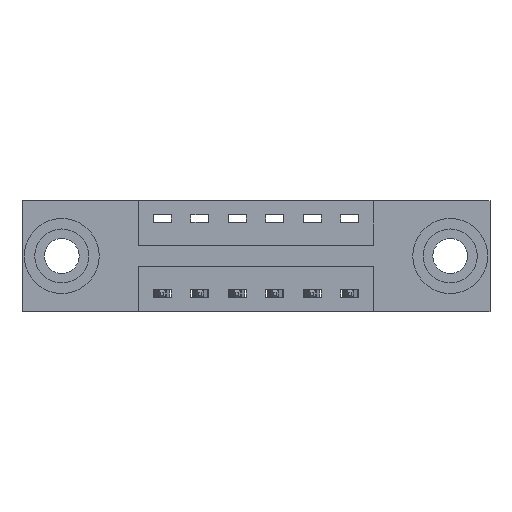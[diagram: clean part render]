
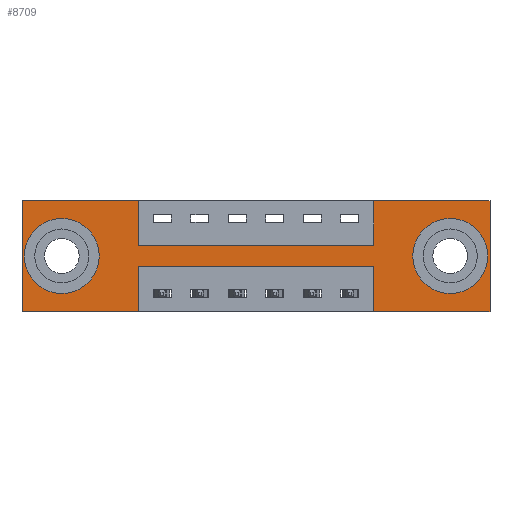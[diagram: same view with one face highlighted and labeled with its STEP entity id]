
A CAD part, front view. The second image highlights one B-rep face of the part: STEP entity #8709.
In plain terms, the highlighted planar face has unit normal (0, -1, 0).
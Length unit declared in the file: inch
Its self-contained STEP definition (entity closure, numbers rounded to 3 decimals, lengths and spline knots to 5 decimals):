
#26 = LINE ( 'NONE', #4180, #5524 ) ;
#77 = EDGE_LOOP ( 'NONE', ( #3163, #3465 ) ) ;
#123 = VERTEX_POINT ( 'NONE', #2344 ) ;
#150 = EDGE_CURVE ( 'NONE', #1095, #9016, #529, .T. ) ;
#191 = CARTESIAN_POINT ( 'NONE',  ( 0., 0., -0.37 ) ) ;
#247 = EDGE_CURVE ( 'NONE', #3096, #1057, #26, .T. ) ;
#474 = CARTESIAN_POINT ( 'NONE',  ( 0.1325, 0., -0.185 ) ) ;
#517 = EDGE_CURVE ( 'NONE', #7520, #5748, #3592, .T. ) ;
#529 = CIRCLE ( 'NONE', #5167, 0.078 ) ;
#539 = ORIENTED_EDGE ( 'NONE', *, *, #517, .F. ) ;
#695 = VECTOR ( 'NONE', #3651, 39.37008 ) ;
#874 = DIRECTION ( 'NONE',  ( 0., 0., 1. ) ) ;
#974 = DIRECTION ( 'NONE',  ( 1., 0., 0. ) ) ;
#1005 = ORIENTED_EDGE ( 'NONE', *, *, #8108, .F. ) ;
#1057 = VERTEX_POINT ( 'NONE', #3721 ) ;
#1066 = DIRECTION ( 'NONE',  ( -1., 0., 0. ) ) ;
#1095 = VERTEX_POINT ( 'NONE', #3238 ) ;
#1107 = LINE ( 'NONE', #4271, #6540 ) ;
#1227 = DIRECTION ( 'NONE',  ( 0., 0., 1. ) ) ;
#1295 = VERTEX_POINT ( 'NONE', #2294 ) ;
#1296 = CARTESIAN_POINT ( 'NONE',  ( 0.1325, 0., -0.263 ) ) ;
#1390 = EDGE_CURVE ( 'NONE', #1295, #7130, #1107, .T. ) ;
#1508 = CIRCLE ( 'NONE', #5842, 0.078 ) ;
#1532 = VERTEX_POINT ( 'NONE', #8157 ) ;
#1543 = CARTESIAN_POINT ( 'NONE',  ( 1.1725, 0., 0. ) ) ;
#1601 = EDGE_CURVE ( 'NONE', #4266, #6499, #2909, .T. ) ;
#1611 = FACE_OUTER_BOUND ( 'NONE', #5340, .T. ) ;
#1749 = EDGE_CURVE ( 'NONE', #1057, #4266, #2249, .T. ) ;
#1754 = AXIS2_PLACEMENT_3D ( 'NONE', #3625, #8518, #4333 ) ;
#1825 = AXIS2_PLACEMENT_3D ( 'NONE', #191, #7342, #3143 ) ;
#1878 = DIRECTION ( 'NONE',  ( 1., 0., 0. ) ) ;
#1910 = CARTESIAN_POINT ( 'NONE',  ( 1.4275, 0., -0.185 ) ) ;
#1961 = VECTOR ( 'NONE', #974, 39.37008 ) ;
#2055 = VERTEX_POINT ( 'NONE', #6461 ) ;
#2122 = VECTOR ( 'NONE', #874, 39.37008 ) ;
#2213 = CARTESIAN_POINT ( 'NONE',  ( 0.3875, 0., -0.22 ) ) ;
#2249 = LINE ( 'NONE', #6686, #6193 ) ;
#2294 = CARTESIAN_POINT ( 'NONE',  ( 0.3875, 0., -0.22 ) ) ;
#2318 = EDGE_CURVE ( 'NONE', #9016, #1095, #2347, .T. ) ;
#2344 = CARTESIAN_POINT ( 'NONE',  ( 0.3875, 0., -0.15 ) ) ;
#2347 = CIRCLE ( 'NONE', #3344, 0.078 ) ;
#2526 = VECTOR ( 'NONE', #1066, 39.37008 ) ;
#2622 = DIRECTION ( 'NONE',  ( 0., 0., -1. ) ) ;
#2624 = EDGE_CURVE ( 'NONE', #1532, #123, #5046, .T. ) ;
#2713 = ORIENTED_EDGE ( 'NONE', *, *, #7315, .F. ) ;
#2909 = LINE ( 'NONE', #4907, #8513 ) ;
#2913 = DIRECTION ( 'NONE',  ( -1., 0., 0. ) ) ;
#2933 = CARTESIAN_POINT ( 'NONE',  ( 0., 0., 0. ) ) ;
#2988 = DIRECTION ( 'NONE',  ( 0., 0., -1. ) ) ;
#3096 = VERTEX_POINT ( 'NONE', #1543 ) ;
#3143 = DIRECTION ( 'NONE',  ( 0., 0., -1. ) ) ;
#3163 = ORIENTED_EDGE ( 'NONE', *, *, #4598, .T. ) ;
#3238 = CARTESIAN_POINT ( 'NONE',  ( 0.1325, 0., -0.107 ) ) ;
#3278 = VECTOR ( 'NONE', #4980, 39.37008 ) ;
#3307 = DIRECTION ( 'NONE',  ( 0., 0., 1. ) ) ;
#3344 = AXIS2_PLACEMENT_3D ( 'NONE', #474, #5439, #1227 ) ;
#3366 = ORIENTED_EDGE ( 'NONE', *, *, #150, .T. ) ;
#3465 = ORIENTED_EDGE ( 'NONE', *, *, #7281, .T. ) ;
#3592 = LINE ( 'NONE', #8836, #6770 ) ;
#3612 = ORIENTED_EDGE ( 'NONE', *, *, #1749, .F. ) ;
#3625 = CARTESIAN_POINT ( 'NONE',  ( 1.4275, 0., -0.185 ) ) ;
#3651 = DIRECTION ( 'NONE',  ( 1., 0., 0. ) ) ;
#3721 = CARTESIAN_POINT ( 'NONE',  ( 1.56, 0., 0. ) ) ;
#3775 = LINE ( 'NONE', #5114, #2122 ) ;
#3810 = CARTESIAN_POINT ( 'NONE',  ( 1.1725, 0., -0.37 ) ) ;
#3862 = ORIENTED_EDGE ( 'NONE', *, *, #9186, .F. ) ;
#4157 = ORIENTED_EDGE ( 'NONE', *, *, #2318, .T. ) ;
#4180 = CARTESIAN_POINT ( 'NONE',  ( 0., 0., 0. ) ) ;
#4266 = VERTEX_POINT ( 'NONE', #4353 ) ;
#4271 = CARTESIAN_POINT ( 'NONE',  ( 0.3875, 0., -0.37 ) ) ;
#4313 = CARTESIAN_POINT ( 'NONE',  ( 1.1725, 0., -0.22 ) ) ;
#4333 = DIRECTION ( 'NONE',  ( 0., 0., -1. ) ) ;
#4353 = CARTESIAN_POINT ( 'NONE',  ( 1.56, 0., -0.37 ) ) ;
#4598 = EDGE_CURVE ( 'NONE', #2055, #6014, #1508, .T. ) ;
#4688 = VERTEX_POINT ( 'NONE', #6932 ) ;
#4744 = VECTOR ( 'NONE', #5171, 39.37008 ) ;
#4834 = CARTESIAN_POINT ( 'NONE',  ( 0.3875, 0., -0.37 ) ) ;
#4858 = VECTOR ( 'NONE', #5798, 39.37008 ) ;
#4907 = CARTESIAN_POINT ( 'NONE',  ( 0., 0., -0.37 ) ) ;
#4967 = EDGE_CURVE ( 'NONE', #123, #4688, #5438, .T. ) ;
#4980 = DIRECTION ( 'NONE',  ( -1., 0., 0. ) ) ;
#5046 = LINE ( 'NONE', #5091, #4858 ) ;
#5091 = CARTESIAN_POINT ( 'NONE',  ( 0.3875, 0., 0. ) ) ;
#5114 = CARTESIAN_POINT ( 'NONE',  ( 1.1725, 0., 0. ) ) ;
#5167 = AXIS2_PLACEMENT_3D ( 'NONE', #7393, #7113, #8454 ) ;
#5171 = DIRECTION ( 'NONE',  ( 0., 0., 1. ) ) ;
#5281 = CARTESIAN_POINT ( 'NONE',  ( 0., 0., -0.37 ) ) ;
#5298 = ORIENTED_EDGE ( 'NONE', *, *, #6175, .F. ) ;
#5321 = FACE_BOUND ( 'NONE', #8372, .T. ) ;
#5340 = EDGE_LOOP ( 'NONE', ( #6370, #3862, #8974, #8254, #3612, #9002, #5298, #6465, #5616, #2713, #539, #1005 ) ) ;
#5438 = LINE ( 'NONE', #5947, #1961 ) ;
#5439 = DIRECTION ( 'NONE',  ( 0., 1., 0. ) ) ;
#5524 = VECTOR ( 'NONE', #1878, 39.37008 ) ;
#5616 = ORIENTED_EDGE ( 'NONE', *, *, #2624, .F. ) ;
#5748 = VERTEX_POINT ( 'NONE', #8158 ) ;
#5798 = DIRECTION ( 'NONE',  ( 0., 0., -1. ) ) ;
#5842 = AXIS2_PLACEMENT_3D ( 'NONE', #1910, #6811, #2622 ) ;
#5867 = PLANE ( 'NONE',  #1825 ) ;
#5947 = CARTESIAN_POINT ( 'NONE',  ( 0.3875, 0., -0.15 ) ) ;
#6004 = LINE ( 'NONE', #5281, #2526 ) ;
#6014 = VERTEX_POINT ( 'NONE', #7666 ) ;
#6175 = EDGE_CURVE ( 'NONE', #4688, #3096, #3775, .T. ) ;
#6193 = VECTOR ( 'NONE', #6698, 39.37008 ) ;
#6367 = LINE ( 'NONE', #2933, #695 ) ;
#6370 = ORIENTED_EDGE ( 'NONE', *, *, #1390, .F. ) ;
#6461 = CARTESIAN_POINT ( 'NONE',  ( 1.4275, 0., -0.107 ) ) ;
#6465 = ORIENTED_EDGE ( 'NONE', *, *, #4967, .F. ) ;
#6499 = VERTEX_POINT ( 'NONE', #7002 ) ;
#6540 = VECTOR ( 'NONE', #2988, 39.37008 ) ;
#6592 = VERTEX_POINT ( 'NONE', #4313 ) ;
#6600 = CIRCLE ( 'NONE', #1754, 0.078 ) ;
#6686 = CARTESIAN_POINT ( 'NONE',  ( 1.56, 0., 0. ) ) ;
#6698 = DIRECTION ( 'NONE',  ( 0., 0., -1. ) ) ;
#6770 = VECTOR ( 'NONE', #3307, 39.37008 ) ;
#6791 = EDGE_CURVE ( 'NONE', #6499, #6592, #8692, .T. ) ;
#6811 = DIRECTION ( 'NONE',  ( 0., 1., 0. ) ) ;
#6932 = CARTESIAN_POINT ( 'NONE',  ( 1.1725, 0., -0.15 ) ) ;
#7002 = CARTESIAN_POINT ( 'NONE',  ( 1.1725, 0., -0.37 ) ) ;
#7113 = DIRECTION ( 'NONE',  ( 0., 1., 0. ) ) ;
#7130 = VERTEX_POINT ( 'NONE', #4834 ) ;
#7281 = EDGE_CURVE ( 'NONE', #6014, #2055, #6600, .T. ) ;
#7315 = EDGE_CURVE ( 'NONE', #5748, #1532, #6367, .T. ) ;
#7342 = DIRECTION ( 'NONE',  ( 0., -1., 0. ) ) ;
#7393 = CARTESIAN_POINT ( 'NONE',  ( 0.1325, 0., -0.185 ) ) ;
#7520 = VERTEX_POINT ( 'NONE', #8044 ) ;
#7666 = CARTESIAN_POINT ( 'NONE',  ( 1.4275, 0., -0.263 ) ) ;
#8044 = CARTESIAN_POINT ( 'NONE',  ( 0., 0., -0.37 ) ) ;
#8108 = EDGE_CURVE ( 'NONE', #7130, #7520, #6004, .T. ) ;
#8157 = CARTESIAN_POINT ( 'NONE',  ( 0.3875, 0., 0. ) ) ;
#8158 = CARTESIAN_POINT ( 'NONE',  ( 0., 0., 0. ) ) ;
#8254 = ORIENTED_EDGE ( 'NONE', *, *, #1601, .F. ) ;
#8372 = EDGE_LOOP ( 'NONE', ( #3366, #4157 ) ) ;
#8454 = DIRECTION ( 'NONE',  ( 0., 0., 1. ) ) ;
#8513 = VECTOR ( 'NONE', #2913, 39.37008 ) ;
#8518 = DIRECTION ( 'NONE',  ( 0., 1., 0. ) ) ;
#8692 = LINE ( 'NONE', #3810, #4744 ) ;
#8709 = ADVANCED_FACE ( 'NONE', ( #9112, #5321, #1611 ), #5867, .T. ) ;
#8836 = CARTESIAN_POINT ( 'NONE',  ( 0., 0., 0. ) ) ;
#8879 = LINE ( 'NONE', #2213, #3278 ) ;
#8974 = ORIENTED_EDGE ( 'NONE', *, *, #6791, .F. ) ;
#9002 = ORIENTED_EDGE ( 'NONE', *, *, #247, .F. ) ;
#9016 = VERTEX_POINT ( 'NONE', #1296 ) ;
#9112 = FACE_BOUND ( 'NONE', #77, .T. ) ;
#9186 = EDGE_CURVE ( 'NONE', #6592, #1295, #8879, .T. ) ;
